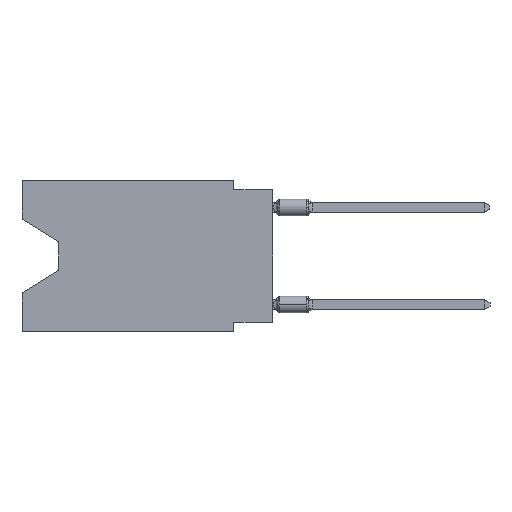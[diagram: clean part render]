
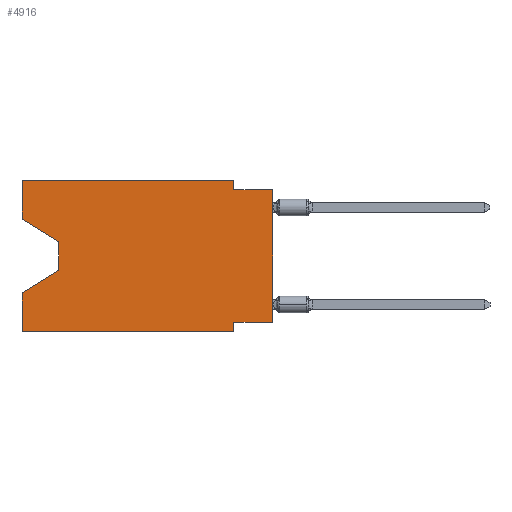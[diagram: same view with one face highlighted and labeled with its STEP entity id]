
A CAD part, left-side view. The second image highlights one B-rep face of the part: STEP entity #4916.
In plain terms, the highlighted planar face has unit normal (-1, 0, 0).
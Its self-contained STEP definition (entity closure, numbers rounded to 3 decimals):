
#64 = LINE ( 'NONE', #7921, #11960 ) ;
#177 = CARTESIAN_POINT ( 'NONE',  ( 0., 16.383, -9.906 ) ) ;
#179 = CARTESIAN_POINT ( 'NONE',  ( 0., 13.97, -4.013 ) ) ;
#306 = ORIENTED_EDGE ( 'NONE', *, *, #8465, .F. ) ;
#437 = ORIENTED_EDGE ( 'NONE', *, *, #11659, .T. ) ;
#444 = CARTESIAN_POINT ( 'NONE',  ( 0., 2.54, -0.635 ) ) ;
#447 = VECTOR ( 'NONE', #12544, 1000. ) ;
#597 = CARTESIAN_POINT ( 'NONE',  ( 0., 16.383, -2.546 ) ) ;
#649 = LINE ( 'NONE', #13965, #7691 ) ;
#736 = VERTEX_POINT ( 'NONE', #3009 ) ;
#747 = CARTESIAN_POINT ( 'NONE',  ( 0., 2.54, -9.906 ) ) ;
#795 = ORIENTED_EDGE ( 'NONE', *, *, #8473, .F. ) ;
#994 = VECTOR ( 'NONE', #8803, 1000. ) ;
#1015 = DIRECTION ( 'NONE',  ( 0., -1., 0. ) ) ;
#1058 = VECTOR ( 'NONE', #9483, 1000. ) ;
#1207 = CARTESIAN_POINT ( 'NONE',  ( 0., 2.54, 0. ) ) ;
#1290 = CARTESIAN_POINT ( 'NONE',  ( 0., 13.97, -4.013 ) ) ;
#1648 = CARTESIAN_POINT ( 'NONE',  ( 0., 16.383, 0. ) ) ;
#1802 = VERTEX_POINT ( 'NONE', #2529 ) ;
#2131 = AXIS2_PLACEMENT_3D ( 'NONE', #4371, #13637, #12069 ) ;
#2152 = EDGE_CURVE ( 'NONE', #8223, #10478, #11306, .T. ) ;
#2529 = CARTESIAN_POINT ( 'NONE',  ( 0., 2.54, 0. ) ) ;
#2918 = DIRECTION ( 'NONE',  ( 0., 0., 1. ) ) ;
#3009 = CARTESIAN_POINT ( 'NONE',  ( 0., 0., -9.271 ) ) ;
#3460 = DIRECTION ( 'NONE',  ( 0., 0., 1. ) ) ;
#3513 = VERTEX_POINT ( 'NONE', #11802 ) ;
#3546 = VECTOR ( 'NONE', #4039, 1000. ) ;
#3665 = EDGE_CURVE ( 'NONE', #1802, #5923, #8920, .T. ) ;
#3867 = EDGE_CURVE ( 'NONE', #7314, #4672, #7108, .T. ) ;
#4039 = DIRECTION ( 'NONE',  ( 0., 0., -1. ) ) ;
#4138 = ORIENTED_EDGE ( 'NONE', *, *, #4738, .T. ) ;
#4274 = CARTESIAN_POINT ( 'NONE',  ( 0., 2.54, -9.906 ) ) ;
#4319 = ORIENTED_EDGE ( 'NONE', *, *, #10793, .F. ) ;
#4371 = CARTESIAN_POINT ( 'NONE',  ( 0., 16.383, 0. ) ) ;
#4634 = ORIENTED_EDGE ( 'NONE', *, *, #8813, .F. ) ;
#4672 = VERTEX_POINT ( 'NONE', #9178 ) ;
#4738 = EDGE_CURVE ( 'NONE', #736, #6573, #649, .T. ) ;
#4916 = ADVANCED_FACE ( 'NONE', ( #10984 ), #11049, .F. ) ;
#5453 = EDGE_CURVE ( 'NONE', #7314, #13168, #8101, .T. ) ;
#5755 = CARTESIAN_POINT ( 'NONE',  ( 0., 0., -9.271 ) ) ;
#5923 = VERTEX_POINT ( 'NONE', #444 ) ;
#6183 = ORIENTED_EDGE ( 'NONE', *, *, #3867, .F. ) ;
#6545 = ORIENTED_EDGE ( 'NONE', *, *, #9102, .F. ) ;
#6573 = VERTEX_POINT ( 'NONE', #14307 ) ;
#6664 = LINE ( 'NONE', #6953, #14221 ) ;
#6953 = CARTESIAN_POINT ( 'NONE',  ( 0., 16.383, 0. ) ) ;
#6979 = DIRECTION ( 'NONE',  ( 0., 0., -1. ) ) ;
#7108 = LINE ( 'NONE', #1648, #11953 ) ;
#7252 = LINE ( 'NONE', #11679, #11905 ) ;
#7314 = VERTEX_POINT ( 'NONE', #11196 ) ;
#7691 = VECTOR ( 'NONE', #2918, 1000. ) ;
#7859 = ORIENTED_EDGE ( 'NONE', *, *, #5453, .T. ) ;
#7921 = CARTESIAN_POINT ( 'NONE',  ( 0., 16.383, 0. ) ) ;
#8010 = EDGE_LOOP ( 'NONE', ( #7859, #8786, #437, #4634, #10762, #6545, #4319, #4138, #795, #11292, #306, #6183 ) ) ;
#8101 = LINE ( 'NONE', #597, #1058 ) ;
#8223 = VERTEX_POINT ( 'NONE', #12443 ) ;
#8413 = DIRECTION ( 'NONE',  ( 0., 0.855, -0.519 ) ) ;
#8465 = EDGE_CURVE ( 'NONE', #4672, #1802, #64, .T. ) ;
#8473 = EDGE_CURVE ( 'NONE', #5923, #6573, #8934, .T. ) ;
#8615 = VERTEX_POINT ( 'NONE', #10252 ) ;
#8786 = ORIENTED_EDGE ( 'NONE', *, *, #12663, .T. ) ;
#8803 = DIRECTION ( 'NONE',  ( 0., 1., 0. ) ) ;
#8813 = EDGE_CURVE ( 'NONE', #8223, #8615, #6664, .T. ) ;
#8920 = LINE ( 'NONE', #1207, #12652 ) ;
#8934 = LINE ( 'NONE', #10987, #14290 ) ;
#9102 = EDGE_CURVE ( 'NONE', #3513, #10478, #10861, .T. ) ;
#9178 = CARTESIAN_POINT ( 'NONE',  ( 0., 16.383, 0. ) ) ;
#9483 = DIRECTION ( 'NONE',  ( 0., -0.855, -0.519 ) ) ;
#9578 = CARTESIAN_POINT ( 'NONE',  ( 0., 13.97, -5.893 ) ) ;
#10252 = CARTESIAN_POINT ( 'NONE',  ( 0., 16.383, -7.36 ) ) ;
#10335 = VERTEX_POINT ( 'NONE', #9578 ) ;
#10478 = VERTEX_POINT ( 'NONE', #4274 ) ;
#10762 = ORIENTED_EDGE ( 'NONE', *, *, #2152, .T. ) ;
#10793 = EDGE_CURVE ( 'NONE', #736, #3513, #12431, .T. ) ;
#10861 = LINE ( 'NONE', #747, #3546 ) ;
#10984 = FACE_OUTER_BOUND ( 'NONE', #8010, .T. ) ;
#10987 = CARTESIAN_POINT ( 'NONE',  ( 0., 0., -0.635 ) ) ;
#11049 = PLANE ( 'NONE',  #2131 ) ;
#11196 = CARTESIAN_POINT ( 'NONE',  ( 0., 16.383, -2.546 ) ) ;
#11292 = ORIENTED_EDGE ( 'NONE', *, *, #3665, .F. ) ;
#11306 = LINE ( 'NONE', #177, #447 ) ;
#11659 = EDGE_CURVE ( 'NONE', #10335, #8615, #7252, .T. ) ;
#11679 = CARTESIAN_POINT ( 'NONE',  ( 0., 13.97, -5.893 ) ) ;
#11802 = CARTESIAN_POINT ( 'NONE',  ( 0., 2.54, -9.271 ) ) ;
#11905 = VECTOR ( 'NONE', #8413, 1000. ) ;
#11953 = VECTOR ( 'NONE', #12694, 1000. ) ;
#11960 = VECTOR ( 'NONE', #14322, 1000. ) ;
#12069 = DIRECTION ( 'NONE',  ( 0., 0., -1. ) ) ;
#12431 = LINE ( 'NONE', #5755, #994 ) ;
#12443 = CARTESIAN_POINT ( 'NONE',  ( 0., 16.383, -9.906 ) ) ;
#12544 = DIRECTION ( 'NONE',  ( 0., -1., 0. ) ) ;
#12652 = VECTOR ( 'NONE', #13568, 1000. ) ;
#12663 = EDGE_CURVE ( 'NONE', #13168, #10335, #13574, .T. ) ;
#12694 = DIRECTION ( 'NONE',  ( 0., 0., 1. ) ) ;
#13168 = VERTEX_POINT ( 'NONE', #179 ) ;
#13568 = DIRECTION ( 'NONE',  ( 0., 0., -1. ) ) ;
#13574 = LINE ( 'NONE', #1290, #13670 ) ;
#13637 = DIRECTION ( 'NONE',  ( 1., 0., 0. ) ) ;
#13670 = VECTOR ( 'NONE', #6979, 1000. ) ;
#13965 = CARTESIAN_POINT ( 'NONE',  ( 0., 0., 0. ) ) ;
#14221 = VECTOR ( 'NONE', #3460, 1000. ) ;
#14290 = VECTOR ( 'NONE', #1015, 1000. ) ;
#14307 = CARTESIAN_POINT ( 'NONE',  ( 0., 0., -0.635 ) ) ;
#14322 = DIRECTION ( 'NONE',  ( 0., -1., 0. ) ) ;
